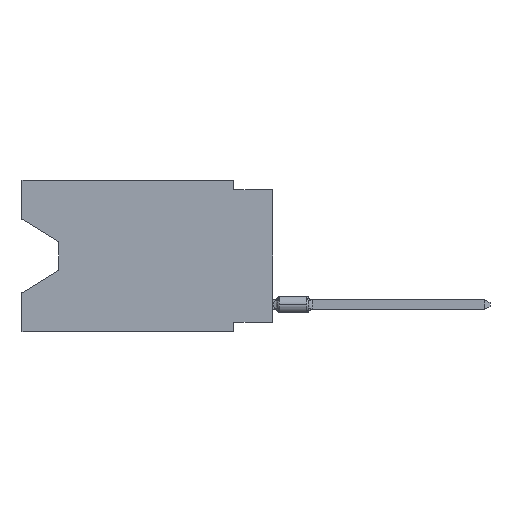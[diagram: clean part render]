
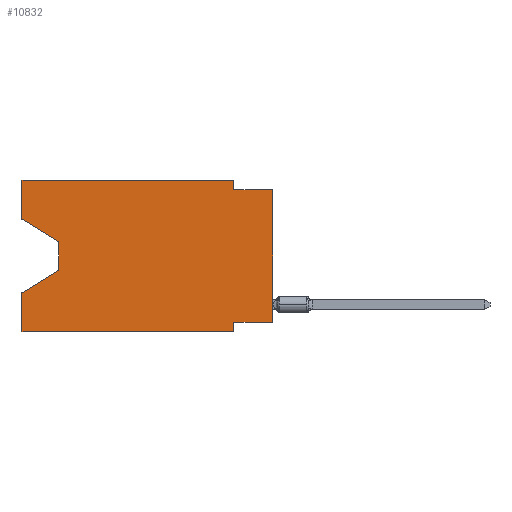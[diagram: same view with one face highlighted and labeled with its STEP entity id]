
A CAD part, left-side view. The second image highlights one B-rep face of the part: STEP entity #10832.
In plain terms, the highlighted planar face has unit normal (-1, 0, 0).
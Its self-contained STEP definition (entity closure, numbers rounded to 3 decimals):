
#91 = EDGE_CURVE ( 'NONE', #18089, #31769, #8321, .T. ) ;
#347 = EDGE_CURVE ( 'NONE', #5138, #14214, #7105, .T. ) ;
#383 = CARTESIAN_POINT ( 'NONE',  ( 0., 2.54, 0. ) ) ;
#435 = LINE ( 'NONE', #615, #22770 ) ;
#615 = CARTESIAN_POINT ( 'NONE',  ( 0., 0., -0.635 ) ) ;
#1093 = VECTOR ( 'NONE', #29613, 1000. ) ;
#1161 = DIRECTION ( 'NONE',  ( 0., 0., -1. ) ) ;
#1949 = EDGE_CURVE ( 'NONE', #20094, #23582, #18470, .T. ) ;
#1974 = LINE ( 'NONE', #22552, #24641 ) ;
#2254 = DIRECTION ( 'NONE',  ( 0., 0., -1. ) ) ;
#2341 = EDGE_LOOP ( 'NONE', ( #24515, #14289, #17389, #13044, #3353, #14713, #28114, #21607, #17769, #33187, #23809, #10141 ) ) ;
#2910 = CARTESIAN_POINT ( 'NONE',  ( 0., 2.54, -9.271 ) ) ;
#3353 = ORIENTED_EDGE ( 'NONE', *, *, #13762, .T. ) ;
#4380 = CARTESIAN_POINT ( 'NONE',  ( 0., 16.383, 0. ) ) ;
#4671 = DIRECTION ( 'NONE',  ( 0., 0., 1. ) ) ;
#5138 = VERTEX_POINT ( 'NONE', #17968 ) ;
#5216 = CARTESIAN_POINT ( 'NONE',  ( 0., 2.54, -0.635 ) ) ;
#6537 = LINE ( 'NONE', #17315, #8578 ) ;
#6693 = DIRECTION ( 'NONE',  ( 0., 1., 0. ) ) ;
#6742 = EDGE_CURVE ( 'NONE', #7163, #11511, #25988, .T. ) ;
#6812 = DIRECTION ( 'NONE',  ( 0., -1., 0. ) ) ;
#7105 = LINE ( 'NONE', #32906, #31592 ) ;
#7146 = CARTESIAN_POINT ( 'NONE',  ( 0., 2.54, -9.906 ) ) ;
#7163 = VERTEX_POINT ( 'NONE', #2910 ) ;
#7437 = CARTESIAN_POINT ( 'NONE',  ( 0., 13.97, -5.893 ) ) ;
#7762 = DIRECTION ( 'NONE',  ( 0., -0.855, -0.519 ) ) ;
#8321 = LINE ( 'NONE', #383, #31290 ) ;
#8534 = VECTOR ( 'NONE', #2254, 1000. ) ;
#8578 = VECTOR ( 'NONE', #6693, 1000. ) ;
#9490 = VERTEX_POINT ( 'NONE', #32879 ) ;
#10141 = ORIENTED_EDGE ( 'NONE', *, *, #27530, .F. ) ;
#10832 = ADVANCED_FACE ( 'NONE', ( #15882 ), #14148, .F. ) ;
#10921 = DIRECTION ( 'NONE',  ( 0., 0., -1. ) ) ;
#11377 = CARTESIAN_POINT ( 'NONE',  ( 0., 13.97, -4.013 ) ) ;
#11511 = VERTEX_POINT ( 'NONE', #21720 ) ;
#11761 = EDGE_CURVE ( 'NONE', #14214, #20487, #13763, .T. ) ;
#12041 = CARTESIAN_POINT ( 'NONE',  ( 0., 16.383, -7.36 ) ) ;
#12196 = AXIS2_PLACEMENT_3D ( 'NONE', #19183, #16046, #1161 ) ;
#13044 = ORIENTED_EDGE ( 'NONE', *, *, #29419, .F. ) ;
#13762 = EDGE_CURVE ( 'NONE', #21135, #11511, #24711, .T. ) ;
#13763 = LINE ( 'NONE', #23732, #27178 ) ;
#14148 = PLANE ( 'NONE',  #12196 ) ;
#14214 = VERTEX_POINT ( 'NONE', #11377 ) ;
#14289 = ORIENTED_EDGE ( 'NONE', *, *, #11761, .T. ) ;
#14427 = VECTOR ( 'NONE', #6812, 1000. ) ;
#14554 = VECTOR ( 'NONE', #33206, 1000. ) ;
#14713 = ORIENTED_EDGE ( 'NONE', *, *, #6742, .F. ) ;
#15882 = FACE_OUTER_BOUND ( 'NONE', #2341, .T. ) ;
#16046 = DIRECTION ( 'NONE',  ( 1., 0., 0. ) ) ;
#16990 = EDGE_CURVE ( 'NONE', #31769, #23582, #435, .T. ) ;
#17187 = LINE ( 'NONE', #4380, #14554 ) ;
#17315 = CARTESIAN_POINT ( 'NONE',  ( 0., 0., -9.271 ) ) ;
#17389 = ORIENTED_EDGE ( 'NONE', *, *, #26176, .T. ) ;
#17769 = ORIENTED_EDGE ( 'NONE', *, *, #16990, .F. ) ;
#17817 = CARTESIAN_POINT ( 'NONE',  ( 0., 2.54, 0. ) ) ;
#17968 = CARTESIAN_POINT ( 'NONE',  ( 0., 16.383, -2.546 ) ) ;
#18089 = VERTEX_POINT ( 'NONE', #17817 ) ;
#18470 = LINE ( 'NONE', #18625, #23062 ) ;
#18625 = CARTESIAN_POINT ( 'NONE',  ( 0., 0., 0. ) ) ;
#19183 = CARTESIAN_POINT ( 'NONE',  ( 0., 16.383, 0. ) ) ;
#19318 = CARTESIAN_POINT ( 'NONE',  ( 0., 16.383, -9.906 ) ) ;
#19342 = CARTESIAN_POINT ( 'NONE',  ( 0., 13.97, -5.893 ) ) ;
#19621 = LINE ( 'NONE', #29920, #14427 ) ;
#19740 = VERTEX_POINT ( 'NONE', #12041 ) ;
#20094 = VERTEX_POINT ( 'NONE', #27639 ) ;
#20487 = VERTEX_POINT ( 'NONE', #7437 ) ;
#21010 = DIRECTION ( 'NONE',  ( 0., -1., 0. ) ) ;
#21133 = DIRECTION ( 'NONE',  ( 0., 0., -1. ) ) ;
#21135 = VERTEX_POINT ( 'NONE', #22225 ) ;
#21607 = ORIENTED_EDGE ( 'NONE', *, *, #1949, .T. ) ;
#21720 = CARTESIAN_POINT ( 'NONE',  ( 0., 2.54, -9.906 ) ) ;
#22225 = CARTESIAN_POINT ( 'NONE',  ( 0., 16.383, -9.906 ) ) ;
#22552 = CARTESIAN_POINT ( 'NONE',  ( 0., 16.383, 0. ) ) ;
#22770 = VECTOR ( 'NONE', #21010, 1000. ) ;
#22978 = CARTESIAN_POINT ( 'NONE',  ( 0., 0., -0.635 ) ) ;
#23062 = VECTOR ( 'NONE', #23704, 1000. ) ;
#23104 = VECTOR ( 'NONE', #24904, 1000. ) ;
#23582 = VERTEX_POINT ( 'NONE', #22978 ) ;
#23704 = DIRECTION ( 'NONE',  ( 0., 0., 1. ) ) ;
#23732 = CARTESIAN_POINT ( 'NONE',  ( 0., 13.97, -4.013 ) ) ;
#23809 = ORIENTED_EDGE ( 'NONE', *, *, #32039, .F. ) ;
#24515 = ORIENTED_EDGE ( 'NONE', *, *, #347, .T. ) ;
#24641 = VECTOR ( 'NONE', #4671, 1000. ) ;
#24711 = LINE ( 'NONE', #19318, #1093 ) ;
#24904 = DIRECTION ( 'NONE',  ( 0., 0.855, -0.519 ) ) ;
#25988 = LINE ( 'NONE', #7146, #8534 ) ;
#26176 = EDGE_CURVE ( 'NONE', #20487, #19740, #32337, .T. ) ;
#26180 = EDGE_CURVE ( 'NONE', #20094, #7163, #6537, .T. ) ;
#27178 = VECTOR ( 'NONE', #10921, 1000. ) ;
#27530 = EDGE_CURVE ( 'NONE', #5138, #9490, #17187, .T. ) ;
#27639 = CARTESIAN_POINT ( 'NONE',  ( 0., 0., -9.271 ) ) ;
#28114 = ORIENTED_EDGE ( 'NONE', *, *, #26180, .F. ) ;
#29419 = EDGE_CURVE ( 'NONE', #21135, #19740, #1974, .T. ) ;
#29613 = DIRECTION ( 'NONE',  ( 0., -1., 0. ) ) ;
#29920 = CARTESIAN_POINT ( 'NONE',  ( 0., 16.383, 0. ) ) ;
#31290 = VECTOR ( 'NONE', #21133, 1000. ) ;
#31592 = VECTOR ( 'NONE', #7762, 1000. ) ;
#31769 = VERTEX_POINT ( 'NONE', #5216 ) ;
#32039 = EDGE_CURVE ( 'NONE', #9490, #18089, #19621, .T. ) ;
#32337 = LINE ( 'NONE', #19342, #23104 ) ;
#32879 = CARTESIAN_POINT ( 'NONE',  ( 0., 16.383, 0. ) ) ;
#32906 = CARTESIAN_POINT ( 'NONE',  ( 0., 16.383, -2.546 ) ) ;
#33187 = ORIENTED_EDGE ( 'NONE', *, *, #91, .F. ) ;
#33206 = DIRECTION ( 'NONE',  ( 0., 0., 1. ) ) ;
